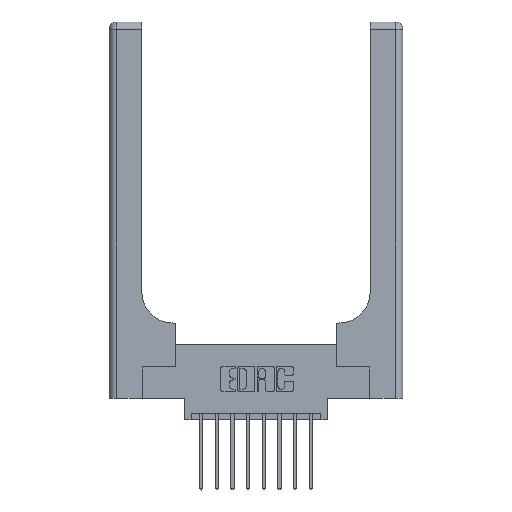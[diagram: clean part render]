
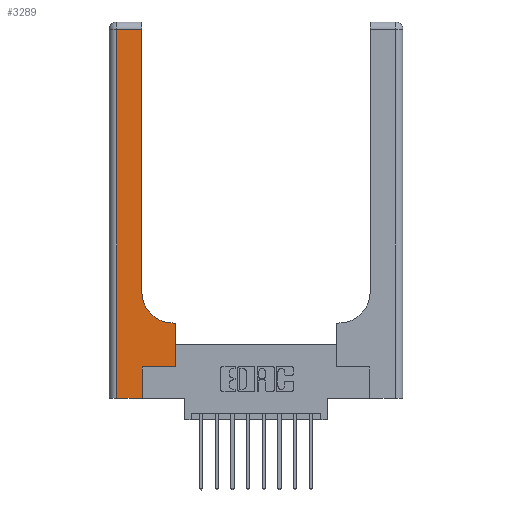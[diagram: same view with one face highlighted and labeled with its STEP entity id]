
A CAD part, top view. The second image highlights one B-rep face of the part: STEP entity #3289.
In plain terms, the highlighted planar face has unit normal (0, 0, 1).
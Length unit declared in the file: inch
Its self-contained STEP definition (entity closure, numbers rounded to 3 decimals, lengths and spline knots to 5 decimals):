
#386 = AXIS2_PLACEMENT_3D ( 'NONE', #9186, #2210, #10392 ) ;
#583 = DIRECTION ( 'NONE',  ( -1., 0., 0. ) ) ;
#913 = LINE ( 'NONE', #1486, #10961 ) ;
#956 = ORIENTED_EDGE ( 'NONE', *, *, #5640, .T. ) ;
#1187 = CIRCLE ( 'NONE', #386, 0.25 ) ;
#1444 = CARTESIAN_POINT ( 'NONE',  ( 0., 2.94, 0.37 ) ) ;
#1486 = CARTESIAN_POINT ( 'NONE',  ( 0.26, 0.6, 0.37 ) ) ;
#1739 = VECTOR ( 'NONE', #9590, 39.37008 ) ;
#1886 = EDGE_CURVE ( 'NONE', #13037, #9658, #913, .T. ) ;
#1911 = CARTESIAN_POINT ( 'NONE',  ( 0.528, 0.25, 0.37 ) ) ;
#1932 = CARTESIAN_POINT ( 'NONE',  ( 0.26, 3., 0.37 ) ) ;
#1965 = VECTOR ( 'NONE', #13651, 39.37008 ) ;
#2086 = CARTESIAN_POINT ( 'NONE',  ( 0.528, 0.6, 0.37 ) ) ;
#2210 = DIRECTION ( 'NONE',  ( 0., 0., -1. ) ) ;
#2259 = ORIENTED_EDGE ( 'NONE', *, *, #7599, .T. ) ;
#2275 = VECTOR ( 'NONE', #5666, 39.37008 ) ;
#2330 = LINE ( 'NONE', #1932, #1965 ) ;
#2344 = CARTESIAN_POINT ( 'NONE',  ( 0.265, 0., 0.37 ) ) ;
#2421 = CARTESIAN_POINT ( 'NONE',  ( 0.06, 2.94, 0.37 ) ) ;
#2585 = LINE ( 'NONE', #5290, #11910 ) ;
#2604 = CARTESIAN_POINT ( 'NONE',  ( 0.265, 0.25, 0.37 ) ) ;
#3089 = DIRECTION ( 'NONE',  ( 0., 1., 0. ) ) ;
#3289 = ADVANCED_FACE ( 'NONE', ( #12394 ), #12236, .F. ) ;
#3556 = VECTOR ( 'NONE', #12914, 39.37008 ) ;
#3844 = EDGE_LOOP ( 'NONE', ( #4253, #956, #14291, #10342, #12824, #2259, #7279, #14202, #9984 ) ) ;
#4120 = DIRECTION ( 'NONE',  ( 0., 1., 0. ) ) ;
#4253 = ORIENTED_EDGE ( 'NONE', *, *, #12962, .T. ) ;
#4649 = LINE ( 'NONE', #10331, #2275 ) ;
#4697 = CARTESIAN_POINT ( 'NONE',  ( 0.26, 0.85, 0.37 ) ) ;
#4709 = CARTESIAN_POINT ( 'NONE',  ( 0.06, 3., 0.37 ) ) ;
#4811 = LINE ( 'NONE', #1444, #7575 ) ;
#5290 = CARTESIAN_POINT ( 'NONE',  ( 0.265, 0., 0.37 ) ) ;
#5463 = EDGE_CURVE ( 'NONE', #9658, #9494, #1187, .T. ) ;
#5538 = VECTOR ( 'NONE', #3089, 39.37008 ) ;
#5556 = EDGE_CURVE ( 'NONE', #10834, #10799, #8648, .T. ) ;
#5640 = EDGE_CURVE ( 'NONE', #9026, #10834, #4811, .T. ) ;
#5666 = DIRECTION ( 'NONE',  ( 1., 0., 0. ) ) ;
#5836 = CARTESIAN_POINT ( 'NONE',  ( 0.06, 0., 0.37 ) ) ;
#6626 = CARTESIAN_POINT ( 'NONE',  ( 0.528, 0.25, 0.37 ) ) ;
#7279 = ORIENTED_EDGE ( 'NONE', *, *, #8493, .T. ) ;
#7485 = CARTESIAN_POINT ( 'NONE',  ( 0.26, 2.94, 0.37 ) ) ;
#7575 = VECTOR ( 'NONE', #8437, 39.37008 ) ;
#7588 = DIRECTION ( 'NONE',  ( 0., 0., -1. ) ) ;
#7599 = EDGE_CURVE ( 'NONE', #14007, #12228, #7959, .T. ) ;
#7735 = CARTESIAN_POINT ( 'NONE',  ( 0.265, 0.25, 0.37 ) ) ;
#7959 = LINE ( 'NONE', #2604, #1739 ) ;
#8437 = DIRECTION ( 'NONE',  ( -1., 0., 0. ) ) ;
#8493 = EDGE_CURVE ( 'NONE', #12228, #13037, #11766, .T. ) ;
#8648 = LINE ( 'NONE', #4709, #3556 ) ;
#9026 = VERTEX_POINT ( 'NONE', #7485 ) ;
#9186 = CARTESIAN_POINT ( 'NONE',  ( 0.51, 0.85, 0.37 ) ) ;
#9494 = VERTEX_POINT ( 'NONE', #4697 ) ;
#9505 = VERTEX_POINT ( 'NONE', #2344 ) ;
#9590 = DIRECTION ( 'NONE',  ( 1., 0., 0. ) ) ;
#9643 = DIRECTION ( 'NONE',  ( -1., 0., 0. ) ) ;
#9658 = VERTEX_POINT ( 'NONE', #13237 ) ;
#9761 = EDGE_CURVE ( 'NONE', #9505, #14007, #2585, .T. ) ;
#9870 = CARTESIAN_POINT ( 'NONE',  ( 0., 3., 0.37 ) ) ;
#9984 = ORIENTED_EDGE ( 'NONE', *, *, #5463, .T. ) ;
#10331 = CARTESIAN_POINT ( 'NONE',  ( 0., 0., 0.37 ) ) ;
#10342 = ORIENTED_EDGE ( 'NONE', *, *, #15115, .T. ) ;
#10392 = DIRECTION ( 'NONE',  ( 1., 0., 0. ) ) ;
#10799 = VERTEX_POINT ( 'NONE', #5836 ) ;
#10834 = VERTEX_POINT ( 'NONE', #2421 ) ;
#10961 = VECTOR ( 'NONE', #9643, 39.37008 ) ;
#11766 = LINE ( 'NONE', #1911, #5538 ) ;
#11817 = AXIS2_PLACEMENT_3D ( 'NONE', #9870, #7588, #583 ) ;
#11910 = VECTOR ( 'NONE', #4120, 39.37008 ) ;
#12228 = VERTEX_POINT ( 'NONE', #6626 ) ;
#12236 = PLANE ( 'NONE',  #11817 ) ;
#12394 = FACE_OUTER_BOUND ( 'NONE', #3844, .T. ) ;
#12824 = ORIENTED_EDGE ( 'NONE', *, *, #9761, .T. ) ;
#12914 = DIRECTION ( 'NONE',  ( 0., -1., 0. ) ) ;
#12962 = EDGE_CURVE ( 'NONE', #9494, #9026, #2330, .T. ) ;
#13037 = VERTEX_POINT ( 'NONE', #2086 ) ;
#13237 = CARTESIAN_POINT ( 'NONE',  ( 0.51, 0.6, 0.37 ) ) ;
#13651 = DIRECTION ( 'NONE',  ( 0., 1., 0. ) ) ;
#14007 = VERTEX_POINT ( 'NONE', #7735 ) ;
#14202 = ORIENTED_EDGE ( 'NONE', *, *, #1886, .T. ) ;
#14291 = ORIENTED_EDGE ( 'NONE', *, *, #5556, .T. ) ;
#15115 = EDGE_CURVE ( 'NONE', #10799, #9505, #4649, .T. ) ;
